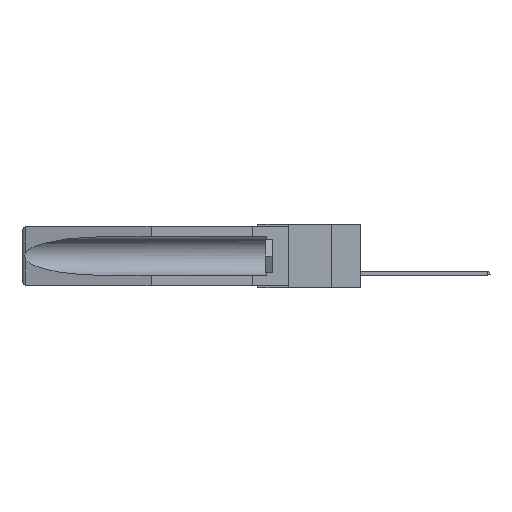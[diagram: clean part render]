
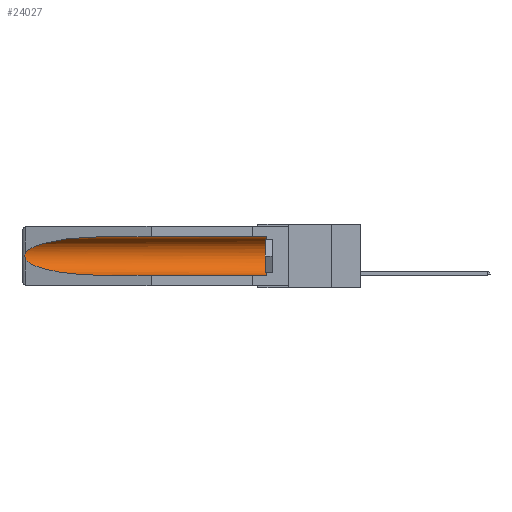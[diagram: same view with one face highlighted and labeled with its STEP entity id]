
A CAD part, left-side view. The second image highlights one B-rep face of the part: STEP entity #24027.
In plain terms, the highlighted cylindrical face has radius 2.857 mm (diameter 5.715 mm), a partial arc.
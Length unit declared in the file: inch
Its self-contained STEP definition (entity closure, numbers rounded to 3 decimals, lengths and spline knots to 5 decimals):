
#33 = CIRCLE ( 'NONE', #4476, 0.1125 ) ;
#254 = ORIENTED_EDGE ( 'NONE', *, *, #16599, .T. ) ;
#644 = DIRECTION ( 'NONE',  ( 0., 1., 0. ) ) ;
#1655 = DIRECTION ( 'NONE',  ( 0., 1., 0. ) ) ;
#2047 = ORIENTED_EDGE ( 'NONE', *, *, #18633, .F. ) ;
#2361 = CARTESIAN_POINT ( 'NONE',  ( 0.2675, 1.53308, -0.16763 ) ) ;
#3988 = LINE ( 'NONE', #11527, #13250 ) ;
#4336 = EDGE_CURVE ( 'NONE', #23620, #17729, #3988, .T. ) ;
#4349 = CARTESIAN_POINT ( 'NONE',  ( 0.155, 1.07973, -0.059 ) ) ;
#4476 = AXIS2_PLACEMENT_3D ( 'NONE', #25908, #17108, #6661 ) ;
#6132 = CARTESIAN_POINT ( 'NONE',  ( 0.26537, 1.52718, -0.14972 ) ) ;
#6661 = DIRECTION ( 'NONE',  ( 0., 0., 1. ) ) ;
#6838 = CARTESIAN_POINT ( 'NONE',  ( 0.2673, 1.5327, -0.16383 ) ) ;
#7868 = CARTESIAN_POINT ( 'NONE',  ( 0.25451, 1.48313, -0.09465 ) ) ;
#8375 = EDGE_CURVE ( 'NONE', #16985, #12648, #17256, .T. ) ;
#8633 = DIRECTION ( 'NONE',  ( 0., 1., 0. ) ) ;
#8742 = AXIS2_PLACEMENT_3D ( 'NONE', #21522, #8633, #23415 ) ;
#8813 = CARTESIAN_POINT ( 'NONE',  ( 0.26654, 1.53092, -0.15636 ) ) ;
#9027 = EDGE_LOOP ( 'NONE', ( #18699, #26011, #13939, #2047, #254, #24392 ) ) ;
#9929 = CARTESIAN_POINT ( 'NONE',  ( 0.26537, 1.52718, -0.19328 ) ) ;
#10009 = CARTESIAN_POINT ( 'NONE',  ( 0.155, 1.07973, -0.059 ) ) ;
#11527 = CARTESIAN_POINT ( 'NONE',  ( 0.155, -0.30754, -0.059 ) ) ;
#12143 = CARTESIAN_POINT ( 'NONE',  ( 0.155, 1.07973, -0.284 ) ) ;
#12187 = EDGE_CURVE ( 'NONE', #17729, #23992, #16576, .T. ) ;
#12224 = LINE ( 'NONE', #22959, #26425 ) ;
#12648 = VERTEX_POINT ( 'NONE', #21856 ) ;
#13250 = VECTOR ( 'NONE', #644, 39.37008 ) ;
#13287 = CYLINDRICAL_SURFACE ( 'NONE', #8742, 0.1125 ) ;
#13435 = VERTEX_POINT ( 'NONE', #18175 ) ;
#13939 = ORIENTED_EDGE ( 'NONE', *, *, #8375, .T. ) ;
#14995 = CARTESIAN_POINT ( 'NONE',  ( 0.26597, 1.5296, -0.19026 ) ) ;
#16576 =( BOUNDED_CURVE ( )  B_SPLINE_CURVE ( 3, ( #10009, #22442, #7868, #27030 ),
 .UNSPECIFIED., .F., .F. ) 
 B_SPLINE_CURVE_WITH_KNOTS ( ( 4, 4 ),
 ( 4.71239, 6.08839 ),
 .UNSPECIFIED. ) 
 CURVE ( )  GEOMETRIC_REPRESENTATION_ITEM ( )  RATIONAL_B_SPLINE_CURVE ( ( 1., 0.848, 0.848, 1. ) ) 
 REPRESENTATION_ITEM ( '' )  );
#16599 = EDGE_CURVE ( 'NONE', #13435, #23620, #33, .T. ) ;
#16985 = VERTEX_POINT ( 'NONE', #18774 ) ;
#17108 = DIRECTION ( 'NONE',  ( 0., -1., 0. ) ) ;
#17256 =( BOUNDED_CURVE ( )  B_SPLINE_CURVE ( 3, ( #9929, #24719, #20476, #12143 ),
 .UNSPECIFIED., .F., .F. ) 
 B_SPLINE_CURVE_WITH_KNOTS ( ( 4, 4 ),
 ( 0.1948, 1.5708 ),
 .UNSPECIFIED. ) 
 CURVE ( )  GEOMETRIC_REPRESENTATION_ITEM ( )  RATIONAL_B_SPLINE_CURVE ( ( 1., 0.848, 0.848, 1. ) ) 
 REPRESENTATION_ITEM ( '' )  );
#17338 = CARTESIAN_POINT ( 'NONE',  ( 0.155, 0.126, -0.059 ) ) ;
#17365 = CARTESIAN_POINT ( 'NONE',  ( 0.26655, 1.53094, -0.18657 ) ) ;
#17459 = CARTESIAN_POINT ( 'NONE',  ( 0.2673, 1.53269, -0.17917 ) ) ;
#17729 = VERTEX_POINT ( 'NONE', #4349 ) ;
#18101 = EDGE_CURVE ( 'NONE', #23992, #16985, #20090, .T. ) ;
#18175 = CARTESIAN_POINT ( 'NONE',  ( 0.155, 0.126, -0.284 ) ) ;
#18633 = EDGE_CURVE ( 'NONE', #13435, #12648, #12224, .T. ) ;
#18699 = ORIENTED_EDGE ( 'NONE', *, *, #12187, .T. ) ;
#18774 = CARTESIAN_POINT ( 'NONE',  ( 0.26537, 1.52718, -0.19328 ) ) ;
#19030 = CARTESIAN_POINT ( 'NONE',  ( 0.26537, 1.52718, -0.14972 ) ) ;
#20090 = B_SPLINE_CURVE_WITH_KNOTS ( 'NONE', 3,
 ( #6132, #20876, #8813, #6838, #2361, #23584, #17459, #17365, #14995, #21696 ),
 .UNSPECIFIED., .F., .F.,
 ( 4, 2, 2, 2, 4 ),
 ( 0., 0.00029, 0.00058, 0.00087, 0.00117 ),
 .UNSPECIFIED. ) ;
#20476 = CARTESIAN_POINT ( 'NONE',  ( 0.21114, 1.30732, -0.284 ) ) ;
#20876 = CARTESIAN_POINT ( 'NONE',  ( 0.26597, 1.52961, -0.15275 ) ) ;
#21522 = CARTESIAN_POINT ( 'NONE',  ( 0.155, -0.30754, -0.1715 ) ) ;
#21696 = CARTESIAN_POINT ( 'NONE',  ( 0.26537, 1.52718, -0.19328 ) ) ;
#21856 = CARTESIAN_POINT ( 'NONE',  ( 0.155, 1.07973, -0.284 ) ) ;
#22442 = CARTESIAN_POINT ( 'NONE',  ( 0.21114, 1.30732, -0.059 ) ) ;
#22959 = CARTESIAN_POINT ( 'NONE',  ( 0.155, -0.30754, -0.284 ) ) ;
#23415 = DIRECTION ( 'NONE',  ( 0., 0., 1. ) ) ;
#23584 = CARTESIAN_POINT ( 'NONE',  ( 0.2675, 1.53308, -0.17534 ) ) ;
#23620 = VERTEX_POINT ( 'NONE', #17338 ) ;
#23992 = VERTEX_POINT ( 'NONE', #19030 ) ;
#24027 = ADVANCED_FACE ( 'NONE', ( #26577 ), #13287, .F. ) ;
#24392 = ORIENTED_EDGE ( 'NONE', *, *, #4336, .T. ) ;
#24719 = CARTESIAN_POINT ( 'NONE',  ( 0.25451, 1.48313, -0.24835 ) ) ;
#25908 = CARTESIAN_POINT ( 'NONE',  ( 0.155, 0.126, -0.1715 ) ) ;
#26011 = ORIENTED_EDGE ( 'NONE', *, *, #18101, .T. ) ;
#26425 = VECTOR ( 'NONE', #1655, 39.37008 ) ;
#26577 = FACE_OUTER_BOUND ( 'NONE', #9027, .T. ) ;
#27030 = CARTESIAN_POINT ( 'NONE',  ( 0.26537, 1.52718, -0.14972 ) ) ;
